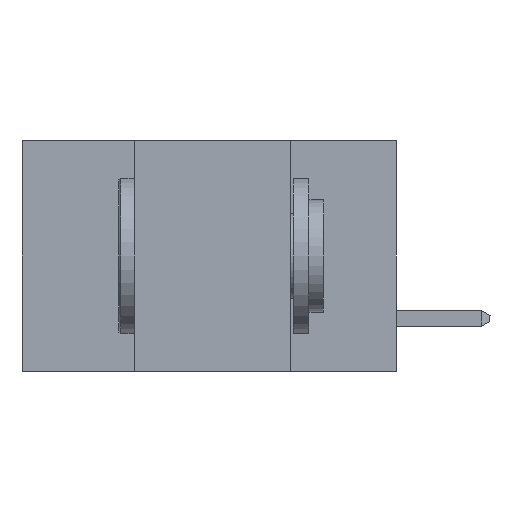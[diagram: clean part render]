
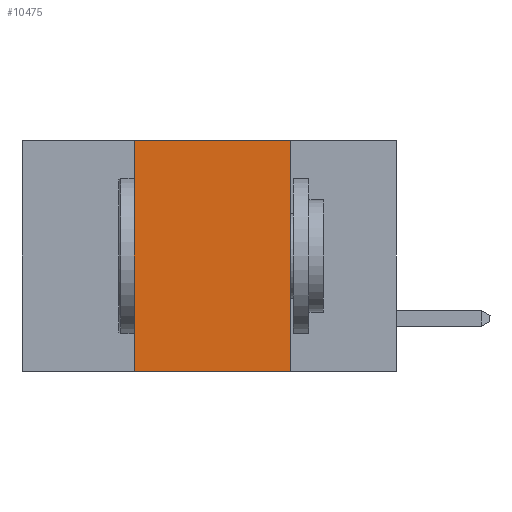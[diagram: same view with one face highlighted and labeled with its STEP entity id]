
A CAD part, left-side view. The second image highlights one B-rep face of the part: STEP entity #10475.
In plain terms, the highlighted planar face has unit normal (-1, 0, 0).
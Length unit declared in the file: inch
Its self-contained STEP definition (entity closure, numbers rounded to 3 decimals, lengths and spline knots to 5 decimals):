
#278 = PLANE ( 'NONE',  #9135 ) ;
#430 = LINE ( 'NONE', #509, #8058 ) ;
#509 = CARTESIAN_POINT ( 'NONE',  ( 0., 0.6, -0.37 ) ) ;
#710 = VERTEX_POINT ( 'NONE', #3156 ) ;
#1037 = EDGE_CURVE ( 'NONE', #5487, #6952, #6758, .T. ) ;
#1196 = CARTESIAN_POINT ( 'NONE',  ( 0., 0.42, -0.37 ) ) ;
#1308 = ORIENTED_EDGE ( 'NONE', *, *, #6388, .F. ) ;
#1348 = DIRECTION ( 'NONE',  ( 0., -1., 0. ) ) ;
#1406 = EDGE_CURVE ( 'NONE', #710, #3318, #430, .T. ) ;
#1482 = ORIENTED_EDGE ( 'NONE', *, *, #1037, .F. ) ;
#1881 = ORIENTED_EDGE ( 'NONE', *, *, #10309, .F. ) ;
#1970 = CARTESIAN_POINT ( 'NONE',  ( 0., 0.17, -0.37 ) ) ;
#2005 = ORIENTED_EDGE ( 'NONE', *, *, #1406, .T. ) ;
#2505 = DIRECTION ( 'NONE',  ( 0., 0., -1. ) ) ;
#2921 = VECTOR ( 'NONE', #8955, 39.37008 ) ;
#3156 = CARTESIAN_POINT ( 'NONE',  ( 0., 0.42, -0.37 ) ) ;
#3318 = VERTEX_POINT ( 'NONE', #8480 ) ;
#3547 = CARTESIAN_POINT ( 'NONE',  ( 0., 0.6, 0. ) ) ;
#4210 = CARTESIAN_POINT ( 'NONE',  ( 0., 0.42, 0. ) ) ;
#5445 = DIRECTION ( 'NONE',  ( 1., 0., 0. ) ) ;
#5487 = VERTEX_POINT ( 'NONE', #4210 ) ;
#5525 = LINE ( 'NONE', #1196, #2921 ) ;
#5657 = DIRECTION ( 'NONE',  ( 0., -1., 0. ) ) ;
#6388 = EDGE_CURVE ( 'NONE', #6952, #3318, #9389, .T. ) ;
#6758 = LINE ( 'NONE', #12184, #8946 ) ;
#6952 = VERTEX_POINT ( 'NONE', #8494 ) ;
#8058 = VECTOR ( 'NONE', #1348, 39.37008 ) ;
#8142 = FACE_OUTER_BOUND ( 'NONE', #9740, .T. ) ;
#8480 = CARTESIAN_POINT ( 'NONE',  ( 0., 0.17, -0.37 ) ) ;
#8494 = CARTESIAN_POINT ( 'NONE',  ( 0., 0.17, 0. ) ) ;
#8717 = DIRECTION ( 'NONE',  ( 0., 0., -1. ) ) ;
#8946 = VECTOR ( 'NONE', #5657, 39.37008 ) ;
#8955 = DIRECTION ( 'NONE',  ( 0., 0., 1. ) ) ;
#9135 = AXIS2_PLACEMENT_3D ( 'NONE', #3547, #5445, #2505 ) ;
#9389 = LINE ( 'NONE', #1970, #12039 ) ;
#9740 = EDGE_LOOP ( 'NONE', ( #1308, #1482, #1881, #2005 ) ) ;
#10309 = EDGE_CURVE ( 'NONE', #710, #5487, #5525, .T. ) ;
#10475 = ADVANCED_FACE ( 'NONE', ( #8142 ), #278, .F. ) ;
#12039 = VECTOR ( 'NONE', #8717, 39.37008 ) ;
#12184 = CARTESIAN_POINT ( 'NONE',  ( 0., 0.6, 0. ) ) ;
